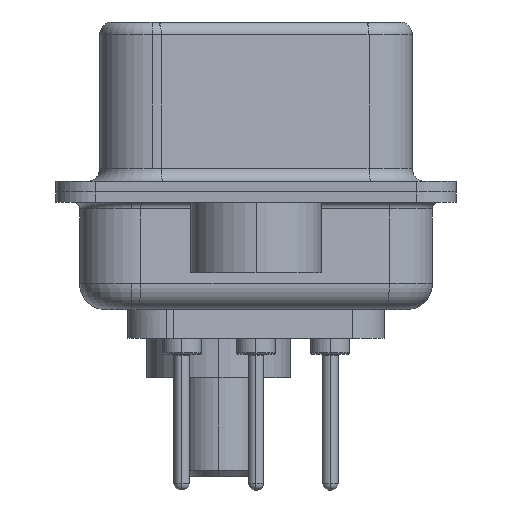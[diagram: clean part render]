
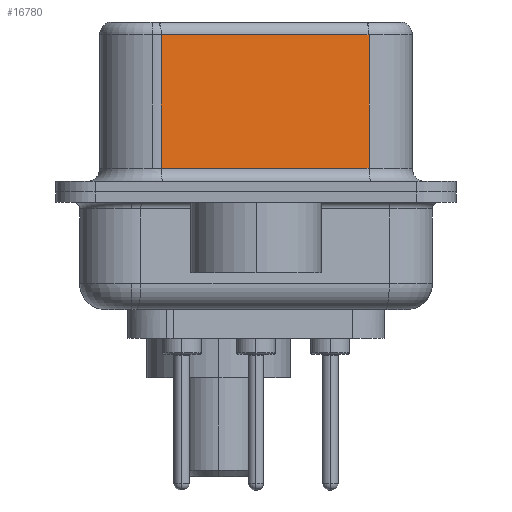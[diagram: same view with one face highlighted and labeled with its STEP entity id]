
A CAD part, left-side view. The second image highlights one B-rep face of the part: STEP entity #16780.
In plain terms, the highlighted planar face has unit normal (-0.985, -0.174, 0).
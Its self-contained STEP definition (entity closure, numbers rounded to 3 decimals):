
#271 = CARTESIAN_POINT ( 'NONE',  ( 3.73, 3.628, 6.52 ) ) ;
#857 = DIRECTION ( 'NONE',  ( 0., 0., -1. ) ) ;
#3120 = CARTESIAN_POINT ( 'NONE',  ( 5.132, -4.322, 0.9 ) ) ;
#3398 = EDGE_CURVE ( 'NONE', #23781, #26939, #17420, .T. ) ;
#4235 = ORIENTED_EDGE ( 'NONE', *, *, #6403, .F. ) ;
#4731 = DIRECTION ( 'NONE',  ( -0.174, 0.985, 0. ) ) ;
#4791 = DIRECTION ( 'NONE',  ( 0., 0., -1. ) ) ;
#5875 = AXIS2_PLACEMENT_3D ( 'NONE', #26127, #17701, #4731 ) ;
#6225 = EDGE_LOOP ( 'NONE', ( #4235, #24554, #26284, #12882 ) ) ;
#6403 = EDGE_CURVE ( 'NONE', #9643, #26939, #22535, .T. ) ;
#6412 = LINE ( 'NONE', #20439, #12202 ) ;
#7099 = CARTESIAN_POINT ( 'NONE',  ( 3.73, 3.628, 0.9 ) ) ;
#9608 = DIRECTION ( 'NONE',  ( -0.174, 0.985, 0. ) ) ;
#9643 = VERTEX_POINT ( 'NONE', #22430 ) ;
#10402 = VERTEX_POINT ( 'NONE', #16022 ) ;
#12202 = VECTOR ( 'NONE', #9608, 1000. ) ;
#12882 = ORIENTED_EDGE ( 'NONE', *, *, #3398, .T. ) ;
#15021 = LINE ( 'NONE', #271, #22210 ) ;
#16022 = CARTESIAN_POINT ( 'NONE',  ( 3.73, 3.628, 6.02 ) ) ;
#16780 = ADVANCED_FACE ( 'NONE', ( #25951 ), #17248, .F. ) ;
#16943 = EDGE_CURVE ( 'NONE', #9643, #10402, #6412, .T. ) ;
#17248 = PLANE ( 'NONE',  #5875 ) ;
#17420 = LINE ( 'NONE', #24985, #22657 ) ;
#17701 = DIRECTION ( 'NONE',  ( 0.985, 0.174, 0. ) ) ;
#18656 = CARTESIAN_POINT ( 'NONE',  ( 5.132, -4.322, 6.52 ) ) ;
#20439 = CARTESIAN_POINT ( 'NONE',  ( 5.132, -4.322, 6.02 ) ) ;
#21849 = VECTOR ( 'NONE', #857, 1000. ) ;
#22017 = EDGE_CURVE ( 'NONE', #10402, #23781, #15021, .T. ) ;
#22210 = VECTOR ( 'NONE', #4791, 1000. ) ;
#22430 = CARTESIAN_POINT ( 'NONE',  ( 5.132, -4.322, 6.02 ) ) ;
#22535 = LINE ( 'NONE', #18656, #21849 ) ;
#22657 = VECTOR ( 'NONE', #24047, 1000. ) ;
#23781 = VERTEX_POINT ( 'NONE', #7099 ) ;
#24047 = DIRECTION ( 'NONE',  ( 0.174, -0.985, 0. ) ) ;
#24554 = ORIENTED_EDGE ( 'NONE', *, *, #16943, .T. ) ;
#24985 = CARTESIAN_POINT ( 'NONE',  ( 5.132, -4.322, 0.9 ) ) ;
#25951 = FACE_OUTER_BOUND ( 'NONE', #6225, .T. ) ;
#26127 = CARTESIAN_POINT ( 'NONE',  ( 5.132, -4.322, 6.52 ) ) ;
#26284 = ORIENTED_EDGE ( 'NONE', *, *, #22017, .T. ) ;
#26939 = VERTEX_POINT ( 'NONE', #3120 ) ;
